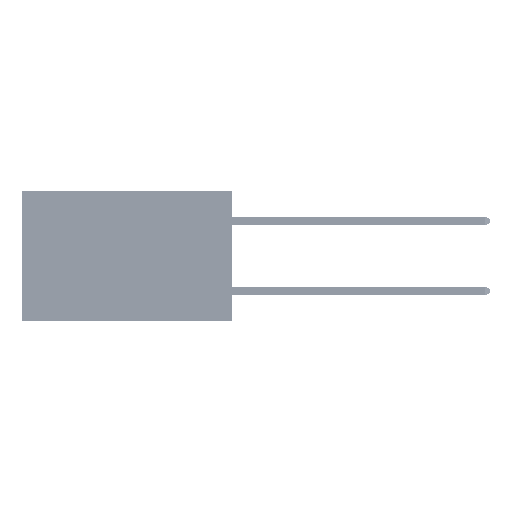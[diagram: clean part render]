
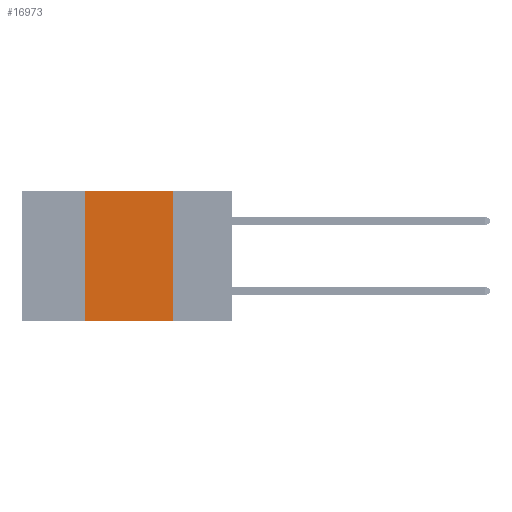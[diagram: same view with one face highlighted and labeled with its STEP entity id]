
A CAD part, left-side view. The second image highlights one B-rep face of the part: STEP entity #16973.
In plain terms, the highlighted planar face has unit normal (-1, 0, 0).
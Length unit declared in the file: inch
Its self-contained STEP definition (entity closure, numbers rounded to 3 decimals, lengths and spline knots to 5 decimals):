
#204 = VERTEX_POINT ( 'NONE', #37847 ) ;
#2962 = VECTOR ( 'NONE', #3385, 39.37008 ) ;
#3327 = VECTOR ( 'NONE', #3364, 39.37008 ) ;
#3364 = DIRECTION ( 'NONE',  ( 0., 0., 1. ) ) ;
#3385 = DIRECTION ( 'NONE',  ( 0., -1., 0. ) ) ;
#3545 = EDGE_CURVE ( 'NONE', #16307, #39461, #29588, .T. ) ;
#6626 = LINE ( 'NONE', #19297, #25744 ) ;
#7229 = DIRECTION ( 'NONE',  ( 0., -1., 0. ) ) ;
#8907 = CARTESIAN_POINT ( 'NONE',  ( 0., 0.6, 0. ) ) ;
#11903 = EDGE_CURVE ( 'NONE', #16307, #204, #13361, .T. ) ;
#12742 = PLANE ( 'NONE',  #17633 ) ;
#12896 = DIRECTION ( 'NONE',  ( 0., 0., -1. ) ) ;
#13361 = LINE ( 'NONE', #15239, #41368 ) ;
#15239 = CARTESIAN_POINT ( 'NONE',  ( 0., 0.6, -0.37 ) ) ;
#15522 = CARTESIAN_POINT ( 'NONE',  ( 0., 0.17, 0. ) ) ;
#16126 = FACE_OUTER_BOUND ( 'NONE', #33768, .T. ) ;
#16307 = VERTEX_POINT ( 'NONE', #27721 ) ;
#16973 = ADVANCED_FACE ( 'NONE', ( #16126 ), #12742, .F. ) ;
#17633 = AXIS2_PLACEMENT_3D ( 'NONE', #8907, #47372, #12896 ) ;
#19297 = CARTESIAN_POINT ( 'NONE',  ( 0., 0.17, 0. ) ) ;
#19684 = CARTESIAN_POINT ( 'NONE',  ( 0., 0.42, 0. ) ) ;
#20882 = VERTEX_POINT ( 'NONE', #15522 ) ;
#25481 = ORIENTED_EDGE ( 'NONE', *, *, #41326, .F. ) ;
#25744 = VECTOR ( 'NONE', #34602, 39.37008 ) ;
#27721 = CARTESIAN_POINT ( 'NONE',  ( 0., 0.42, -0.37 ) ) ;
#28426 = ORIENTED_EDGE ( 'NONE', *, *, #11903, .T. ) ;
#29588 = LINE ( 'NONE', #45681, #3327 ) ;
#32603 = ORIENTED_EDGE ( 'NONE', *, *, #3545, .F. ) ;
#33768 = EDGE_LOOP ( 'NONE', ( #25481, #42338, #32603, #28426 ) ) ;
#34602 = DIRECTION ( 'NONE',  ( 0., 0., -1. ) ) ;
#36424 = LINE ( 'NONE', #45380, #2962 ) ;
#37847 = CARTESIAN_POINT ( 'NONE',  ( 0., 0.17, -0.37 ) ) ;
#39461 = VERTEX_POINT ( 'NONE', #19684 ) ;
#41326 = EDGE_CURVE ( 'NONE', #20882, #204, #6626, .T. ) ;
#41368 = VECTOR ( 'NONE', #7229, 39.37008 ) ;
#41758 = EDGE_CURVE ( 'NONE', #39461, #20882, #36424, .T. ) ;
#42338 = ORIENTED_EDGE ( 'NONE', *, *, #41758, .F. ) ;
#45380 = CARTESIAN_POINT ( 'NONE',  ( 0., 0.6, 0. ) ) ;
#45681 = CARTESIAN_POINT ( 'NONE',  ( 0., 0.42, 0. ) ) ;
#47372 = DIRECTION ( 'NONE',  ( 1., 0., 0. ) ) ;
